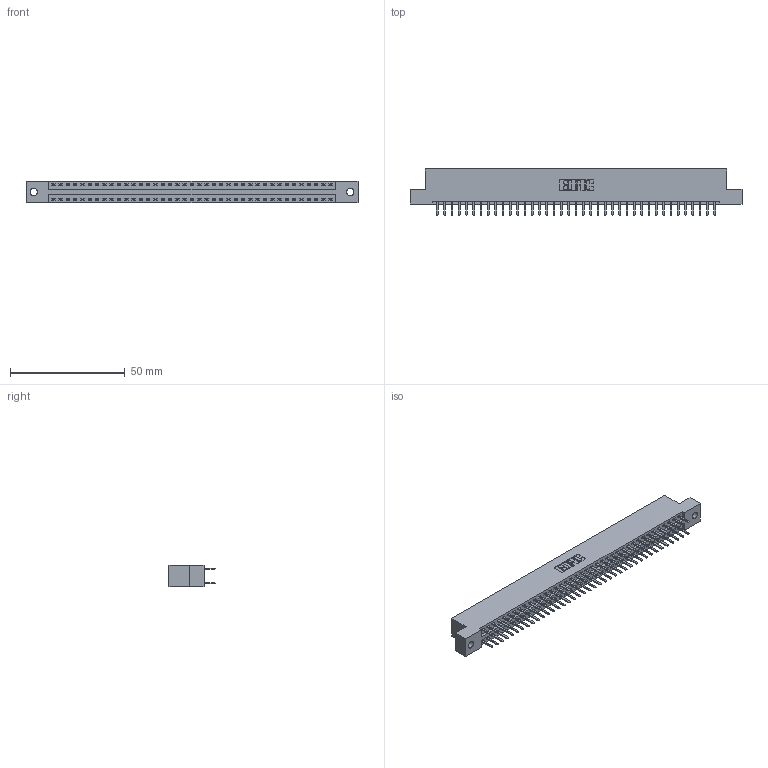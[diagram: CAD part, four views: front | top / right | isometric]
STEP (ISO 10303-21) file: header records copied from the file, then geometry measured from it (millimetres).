
FILE_DESCRIPTION (( 'STEP AP203' ), '1' );
FILE_NAME ('396-078-520-202.STEP', '2018-09-09T14:58:09', ( '' ), ( '' ), 'SwSTEP 2.0', 'SolidWorks 2016', '' );
FILE_SCHEMA (( 'CONFIG_CONTROL_DESIGN' ));
Length unit declared in the file: inch
Products named in the file (3): 346 Part_Flush Mounting Lugs - 0.128 Dia; 345-292-001_345-293-120; 396-078-520-202
Assembly tree (79 placements, depth 2):
  396-078-520-202
    346 Part_Flush Mounting Lugs - 0.128 Dia
    345-292-001_345-293-120  x78
Bounding box: 144.4 x 20.02 x 9.4 mm (x, y, z)
Volume: 13986.4 mm3; surface area: 18828.5 mm2
Topology: 79 solids, 79 shells, 4490 faces, 13043 edges, 8486 vertices
Faces by surface type: plane 2962, cylinder 1528
Entity records: 25973 total; most frequent: CARTESIAN_POINT 4296, ORIENTED_EDGE 4218, DIRECTION 3825, EDGE_CURVE 2109, VECTOR 1817, LINE 1817, VERTEX_POINT 1402, AXIS2_PLACEMENT_3D 1004
